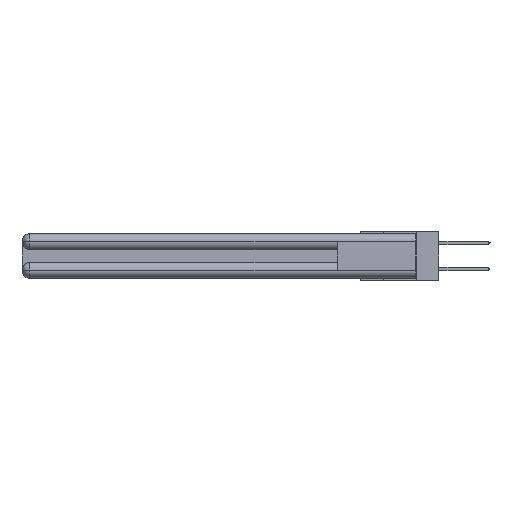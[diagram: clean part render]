
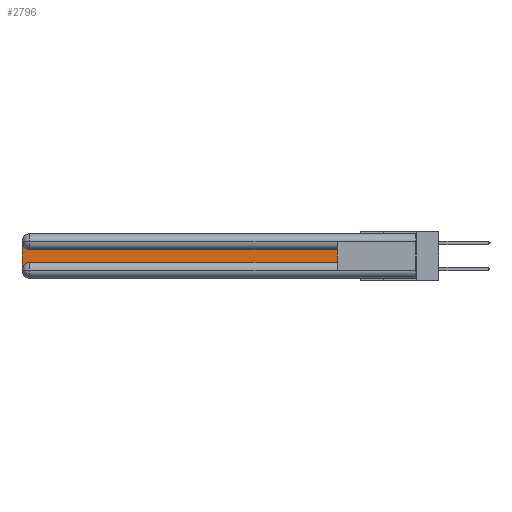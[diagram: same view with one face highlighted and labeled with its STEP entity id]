
A CAD part, left-side view. The second image highlights one B-rep face of the part: STEP entity #2796.
In plain terms, the highlighted planar face has unit normal (-1, 0, 0).
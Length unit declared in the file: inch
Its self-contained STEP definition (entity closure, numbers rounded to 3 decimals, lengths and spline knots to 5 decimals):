
#115 = ORIENTED_EDGE ( 'NONE', *, *, #17460, .T. ) ;
#275 = FACE_OUTER_BOUND ( 'NONE', #22648, .T. ) ;
#957 = DIRECTION ( 'NONE',  ( 0., 0., -1. ) ) ;
#1280 = CARTESIAN_POINT ( 'NONE',  ( 0.075, 3., -0.1225 ) ) ;
#2796 = ADVANCED_FACE ( 'NONE', ( #275 ), #12708, .F. ) ;
#3148 = CARTESIAN_POINT ( 'NONE',  ( 0.075, 2.94, -0.2175 ) ) ;
#3438 = CARTESIAN_POINT ( 'NONE',  ( 0.075, 0.6, -0.2175 ) ) ;
#3754 = CARTESIAN_POINT ( 'NONE',  ( 0.075, 2.94, -0.0625 ) ) ;
#4263 = DIRECTION ( 'NONE',  ( 0., 0., 1. ) ) ;
#5646 = CARTESIAN_POINT ( 'NONE',  ( 0.075, 2.94, -0.2775 ) ) ;
#5702 = DIRECTION ( 'NONE',  ( 0., -1., 0. ) ) ;
#6478 = VECTOR ( 'NONE', #5702, 39.37008 ) ;
#6991 = VERTEX_POINT ( 'NONE', #22594 ) ;
#7292 = CARTESIAN_POINT ( 'NONE',  ( 0.075, 0.6, -0.1225 ) ) ;
#9242 = ORIENTED_EDGE ( 'NONE', *, *, #15340, .T. ) ;
#9413 = CIRCLE ( 'NONE', #11377, 0.06 ) ;
#9865 = VECTOR ( 'NONE', #29759, 39.37008 ) ;
#11377 = AXIS2_PLACEMENT_3D ( 'NONE', #5646, #19144, #22075 ) ;
#11936 = AXIS2_PLACEMENT_3D ( 'NONE', #3754, #15013, #957 ) ;
#12708 = PLANE ( 'NONE',  #23601 ) ;
#13326 = ORIENTED_EDGE ( 'NONE', *, *, #34630, .T. ) ;
#14948 = VERTEX_POINT ( 'NONE', #34915 ) ;
#15013 = DIRECTION ( 'NONE',  ( 1., 0., 0. ) ) ;
#15340 = EDGE_CURVE ( 'NONE', #26088, #34617, #27811, .T. ) ;
#16823 = VERTEX_POINT ( 'NONE', #27794 ) ;
#17349 = DIRECTION ( 'NONE',  ( 0., 0., -1. ) ) ;
#17460 = EDGE_CURVE ( 'NONE', #26729, #16823, #33744, .T. ) ;
#19144 = DIRECTION ( 'NONE',  ( 1., 0., 0. ) ) ;
#19384 = ORIENTED_EDGE ( 'NONE', *, *, #31850, .T. ) ;
#20032 = CARTESIAN_POINT ( 'NONE',  ( 0.075, 0.6, -0.2175 ) ) ;
#22075 = DIRECTION ( 'NONE',  ( 0., 0., -1. ) ) ;
#22249 = ORIENTED_EDGE ( 'NONE', *, *, #27212, .T. ) ;
#22594 = CARTESIAN_POINT ( 'NONE',  ( 0.075, 0.6, -0.1225 ) ) ;
#22648 = EDGE_LOOP ( 'NONE', ( #19384, #115, #22848, #13326, #9242, #22249 ) ) ;
#22848 = ORIENTED_EDGE ( 'NONE', *, *, #26101, .T. ) ;
#22931 = LINE ( 'NONE', #7292, #9865 ) ;
#23601 = AXIS2_PLACEMENT_3D ( 'NONE', #1280, #34580, #23658 ) ;
#23658 = DIRECTION ( 'NONE',  ( 0., 0., -1. ) ) ;
#23990 = CARTESIAN_POINT ( 'NONE',  ( 0.075, 2.94, -0.1225 ) ) ;
#26088 = VERTEX_POINT ( 'NONE', #3148 ) ;
#26101 = EDGE_CURVE ( 'NONE', #16823, #14948, #34208, .T. ) ;
#26729 = VERTEX_POINT ( 'NONE', #23990 ) ;
#26835 = VECTOR ( 'NONE', #17349, 39.37008 ) ;
#27212 = EDGE_CURVE ( 'NONE', #34617, #6991, #30663, .T. ) ;
#27794 = CARTESIAN_POINT ( 'NONE',  ( 0.075, 3., -0.0625 ) ) ;
#27811 = LINE ( 'NONE', #20032, #6478 ) ;
#28393 = CARTESIAN_POINT ( 'NONE',  ( 0.075, 3., -0.2175 ) ) ;
#29759 = DIRECTION ( 'NONE',  ( 0., 1., 0. ) ) ;
#30275 = VECTOR ( 'NONE', #4263, 39.37008 ) ;
#30318 = CARTESIAN_POINT ( 'NONE',  ( 0.075, 0.6, -0.2175 ) ) ;
#30663 = LINE ( 'NONE', #3438, #30275 ) ;
#31850 = EDGE_CURVE ( 'NONE', #6991, #26729, #22931, .T. ) ;
#33744 = CIRCLE ( 'NONE', #11936, 0.06 ) ;
#34208 = LINE ( 'NONE', #28393, #26835 ) ;
#34580 = DIRECTION ( 'NONE',  ( 1., 0., 0. ) ) ;
#34617 = VERTEX_POINT ( 'NONE', #30318 ) ;
#34630 = EDGE_CURVE ( 'NONE', #14948, #26088, #9413, .T. ) ;
#34915 = CARTESIAN_POINT ( 'NONE',  ( 0.075, 3., -0.2775 ) ) ;
